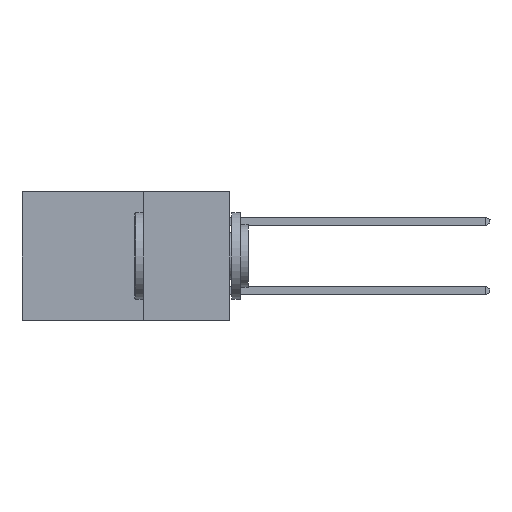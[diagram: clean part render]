
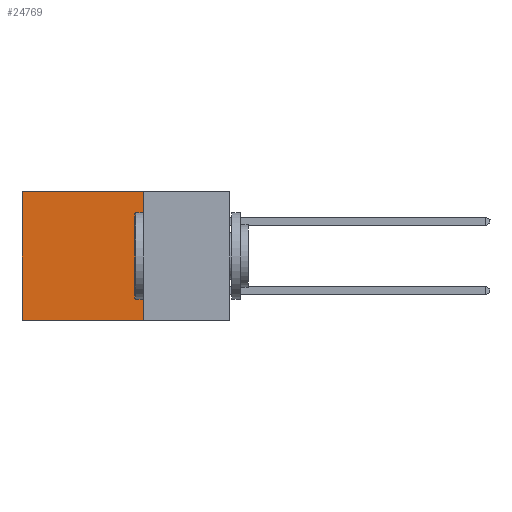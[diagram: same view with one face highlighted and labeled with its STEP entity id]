
A CAD part, left-side view. The second image highlights one B-rep face of the part: STEP entity #24769.
In plain terms, the highlighted planar face has unit normal (-1, 0, 0).
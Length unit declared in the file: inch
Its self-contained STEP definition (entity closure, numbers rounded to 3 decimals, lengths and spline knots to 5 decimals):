
#1364 = CARTESIAN_POINT ( 'NONE',  ( 0.2615, 0.25, 0. ) ) ;
#1871 = DIRECTION ( 'NONE',  ( 0., 1., 0. ) ) ;
#2180 = CARTESIAN_POINT ( 'NONE',  ( 0.2615, 0.6, 0. ) ) ;
#4341 = VERTEX_POINT ( 'NONE', #16779 ) ;
#5137 = DIRECTION ( 'NONE',  ( 0., 0., -1. ) ) ;
#5336 = VERTEX_POINT ( 'NONE', #2180 ) ;
#5697 = DIRECTION ( 'NONE',  ( 0., 0., -1. ) ) ;
#5740 = VERTEX_POINT ( 'NONE', #5819 ) ;
#5819 = CARTESIAN_POINT ( 'NONE',  ( 0.2615, 0.25, -0.37 ) ) ;
#6728 = VECTOR ( 'NONE', #26201, 39.37008 ) ;
#7382 = PLANE ( 'NONE',  #11658 ) ;
#7941 = LINE ( 'NONE', #20569, #25820 ) ;
#8175 = ORIENTED_EDGE ( 'NONE', *, *, #18552, .F. ) ;
#8319 = LINE ( 'NONE', #23702, #20015 ) ;
#8783 = LINE ( 'NONE', #15253, #20578 ) ;
#11185 = ORIENTED_EDGE ( 'NONE', *, *, #19132, .T. ) ;
#11189 = CARTESIAN_POINT ( 'NONE',  ( 0.2615, 0.25, -0.37 ) ) ;
#11658 = AXIS2_PLACEMENT_3D ( 'NONE', #11189, #15955, #5137 ) ;
#13293 = FACE_OUTER_BOUND ( 'NONE', #15189, .T. ) ;
#15189 = EDGE_LOOP ( 'NONE', ( #11185, #8175, #17430, #21092 ) ) ;
#15253 = CARTESIAN_POINT ( 'NONE',  ( 0.2615, 0.25, 0. ) ) ;
#15955 = DIRECTION ( 'NONE',  ( 1., 0., 0. ) ) ;
#16086 = VERTEX_POINT ( 'NONE', #1364 ) ;
#16528 = EDGE_CURVE ( 'NONE', #16086, #5336, #8783, .T. ) ;
#16779 = CARTESIAN_POINT ( 'NONE',  ( 0.2615, 0.6, -0.37 ) ) ;
#17430 = ORIENTED_EDGE ( 'NONE', *, *, #26508, .F. ) ;
#17521 = CARTESIAN_POINT ( 'NONE',  ( 0.2615, 0.25, -0.37 ) ) ;
#18552 = EDGE_CURVE ( 'NONE', #5740, #4341, #8319, .T. ) ;
#19132 = EDGE_CURVE ( 'NONE', #5336, #4341, #7941, .T. ) ;
#20015 = VECTOR ( 'NONE', #1871, 39.37008 ) ;
#20569 = CARTESIAN_POINT ( 'NONE',  ( 0.2615, 0.6, -0.37 ) ) ;
#20578 = VECTOR ( 'NONE', #23799, 39.37008 ) ;
#21092 = ORIENTED_EDGE ( 'NONE', *, *, #16528, .T. ) ;
#21572 = LINE ( 'NONE', #17521, #6728 ) ;
#23702 = CARTESIAN_POINT ( 'NONE',  ( 0.2615, 0.25, -0.37 ) ) ;
#23799 = DIRECTION ( 'NONE',  ( 0., 1., 0. ) ) ;
#24769 = ADVANCED_FACE ( 'NONE', ( #13293 ), #7382, .F. ) ;
#25820 = VECTOR ( 'NONE', #5697, 39.37008 ) ;
#26201 = DIRECTION ( 'NONE',  ( 0., 0., -1. ) ) ;
#26508 = EDGE_CURVE ( 'NONE', #16086, #5740, #21572, .T. ) ;
